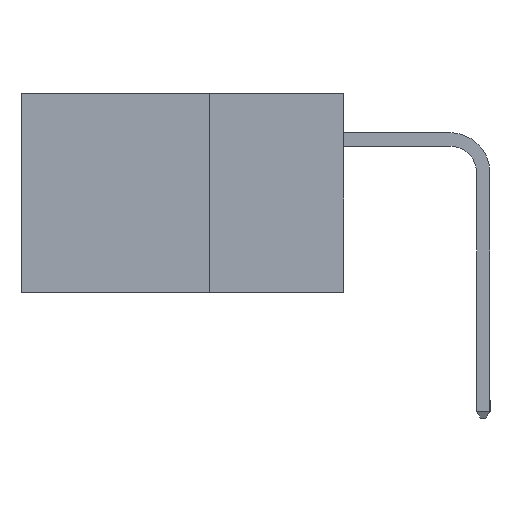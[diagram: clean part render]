
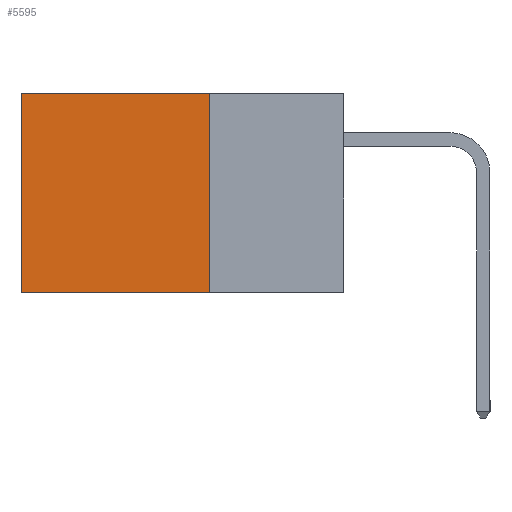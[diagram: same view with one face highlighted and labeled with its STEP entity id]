
A CAD part, left-side view. The second image highlights one B-rep face of the part: STEP entity #5595.
In plain terms, the highlighted planar face has unit normal (-1, 0, 0).
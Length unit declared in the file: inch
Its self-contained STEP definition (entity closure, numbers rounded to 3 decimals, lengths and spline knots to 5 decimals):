
#4 = VERTEX_POINT ( 'NONE', #1946 ) ;
#336 = LINE ( 'NONE', #2253, #2965 ) ;
#428 = ORIENTED_EDGE ( 'NONE', *, *, #4317, .T. ) ;
#476 = ORIENTED_EDGE ( 'NONE', *, *, #4119, .F. ) ;
#496 = ORIENTED_EDGE ( 'NONE', *, *, #9474, .F. ) ;
#508 = ORIENTED_EDGE ( 'NONE', *, *, #4243, .T. ) ;
#705 = VERTEX_POINT ( 'NONE', #5067 ) ;
#789 = DIRECTION ( 'NONE',  ( 0., 0., -1. ) ) ;
#821 = DIRECTION ( 'NONE',  ( 1., 0., 0. ) ) ;
#849 = CARTESIAN_POINT ( 'NONE',  ( 0.2615, 0.25, -0.37 ) ) ;
#881 = PLANE ( 'NONE',  #1303 ) ;
#1303 = AXIS2_PLACEMENT_3D ( 'NONE', #849, #821, #789 ) ;
#1694 = CARTESIAN_POINT ( 'NONE',  ( 0.2615, 0.25, 0. ) ) ;
#1934 = DIRECTION ( 'NONE',  ( 0., 1., 0. ) ) ;
#1946 = CARTESIAN_POINT ( 'NONE',  ( 0.2615, 0.25, -0.37 ) ) ;
#2253 = CARTESIAN_POINT ( 'NONE',  ( 0.2615, 0.25, -0.37 ) ) ;
#2965 = VECTOR ( 'NONE', #1934, 39.37008 ) ;
#3145 = FACE_OUTER_BOUND ( 'NONE', #5022, .T. ) ;
#4119 = EDGE_CURVE ( 'NONE', #4, #9205, #336, .T. ) ;
#4243 = EDGE_CURVE ( 'NONE', #9232, #705, #7464, .T. ) ;
#4317 = EDGE_CURVE ( 'NONE', #705, #9205, #11254, .T. ) ;
#5022 = EDGE_LOOP ( 'NONE', ( #428, #476, #496, #508 ) ) ;
#5067 = CARTESIAN_POINT ( 'NONE',  ( 0.2615, 0.6, 0. ) ) ;
#5308 = VECTOR ( 'NONE', #10817, 39.37008 ) ;
#5595 = ADVANCED_FACE ( 'NONE', ( #3145 ), #881, .F. ) ;
#5609 = DIRECTION ( 'NONE',  ( 0., 0., -1. ) ) ;
#6233 = VECTOR ( 'NONE', #5609, 39.37008 ) ;
#7464 = LINE ( 'NONE', #10673, #5308 ) ;
#9043 = VECTOR ( 'NONE', #10273, 39.37008 ) ;
#9205 = VERTEX_POINT ( 'NONE', #9359 ) ;
#9232 = VERTEX_POINT ( 'NONE', #1694 ) ;
#9359 = CARTESIAN_POINT ( 'NONE',  ( 0.2615, 0.6, -0.37 ) ) ;
#9474 = EDGE_CURVE ( 'NONE', #9232, #4, #10257, .T. ) ;
#9645 = CARTESIAN_POINT ( 'NONE',  ( 0.2615, 0.25, -0.37 ) ) ;
#10257 = LINE ( 'NONE', #9645, #6233 ) ;
#10264 = CARTESIAN_POINT ( 'NONE',  ( 0.2615, 0.6, -0.37 ) ) ;
#10273 = DIRECTION ( 'NONE',  ( 0., 0., -1. ) ) ;
#10673 = CARTESIAN_POINT ( 'NONE',  ( 0.2615, 0.25, 0. ) ) ;
#10817 = DIRECTION ( 'NONE',  ( 0., 1., 0. ) ) ;
#11254 = LINE ( 'NONE', #10264, #9043 ) ;
